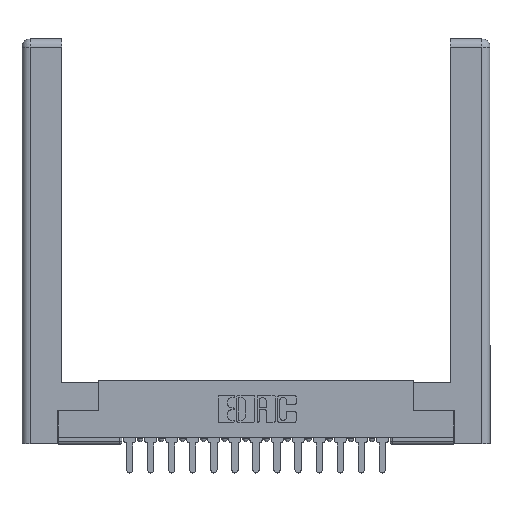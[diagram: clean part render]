
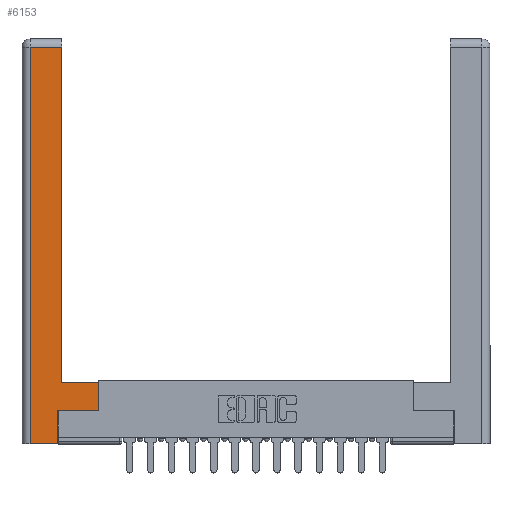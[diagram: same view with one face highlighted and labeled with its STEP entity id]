
A CAD part, top view. The second image highlights one B-rep face of the part: STEP entity #6153.
In plain terms, the highlighted planar face has unit normal (0, 0, 1).
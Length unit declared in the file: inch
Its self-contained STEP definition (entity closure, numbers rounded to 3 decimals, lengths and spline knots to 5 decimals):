
#14 = ORIENTED_EDGE ( 'NONE', *, *, #15030, .T. ) ;
#249 = DIRECTION ( 'NONE',  ( 0., 1., 0. ) ) ;
#354 = CARTESIAN_POINT ( 'NONE',  ( 0.565, 0.245, 0. ) ) ;
#395 = ORIENTED_EDGE ( 'NONE', *, *, #15939, .T. ) ;
#446 = PLANE ( 'NONE',  #3961 ) ;
#534 = DIRECTION ( 'NONE',  ( 0., 0., -1. ) ) ;
#678 = ORIENTED_EDGE ( 'NONE', *, *, #12717, .T. ) ;
#901 = ORIENTED_EDGE ( 'NONE', *, *, #13060, .T. ) ;
#1120 = DIRECTION ( 'NONE',  ( -1., 0., 0. ) ) ;
#1515 = DIRECTION ( 'NONE',  ( 0., 1., 0. ) ) ;
#1787 = FACE_OUTER_BOUND ( 'NONE', #15065, .T. ) ;
#2013 = CARTESIAN_POINT ( 'NONE',  ( 0.295, 3., 0. ) ) ;
#2034 = VERTEX_POINT ( 'NONE', #11718 ) ;
#2072 = CARTESIAN_POINT ( 'NONE',  ( 0.265, 0.245, 0. ) ) ;
#2492 = DIRECTION ( 'NONE',  ( 1., 0., 0. ) ) ;
#2724 = DIRECTION ( 'NONE',  ( -1., 0., 0. ) ) ;
#3560 = VERTEX_POINT ( 'NONE', #7388 ) ;
#3961 = AXIS2_PLACEMENT_3D ( 'NONE', #12844, #534, #8792 ) ;
#4356 = DIRECTION ( 'NONE',  ( 0., 1., 0. ) ) ;
#4361 = EDGE_CURVE ( 'NONE', #13816, #15990, #12673, .T. ) ;
#4656 = VECTOR ( 'NONE', #7862, 39.37008 ) ;
#4718 = CARTESIAN_POINT ( 'NONE',  ( 0.0615, 2.94, 0. ) ) ;
#5055 = LINE ( 'NONE', #14759, #6821 ) ;
#5098 = CARTESIAN_POINT ( 'NONE',  ( 0.565, 0.245, 0. ) ) ;
#5259 = CARTESIAN_POINT ( 'NONE',  ( 0.265, 0., 0. ) ) ;
#5339 = VERTEX_POINT ( 'NONE', #2072 ) ;
#6153 = ADVANCED_FACE ( 'NONE', ( #1787 ), #446, .F. ) ;
#6733 = LINE ( 'NONE', #5098, #16855 ) ;
#6821 = VECTOR ( 'NONE', #1120, 39.37008 ) ;
#7144 = ORIENTED_EDGE ( 'NONE', *, *, #4361, .T. ) ;
#7369 = CARTESIAN_POINT ( 'NONE',  ( 0.265, 0., 0. ) ) ;
#7388 = CARTESIAN_POINT ( 'NONE',  ( 0.295, 0.45, 0. ) ) ;
#7862 = DIRECTION ( 'NONE',  ( 1., 0., 0. ) ) ;
#7930 = LINE ( 'NONE', #8114, #17191 ) ;
#7995 = EDGE_CURVE ( 'NONE', #14933, #5339, #15332, .T. ) ;
#8114 = CARTESIAN_POINT ( 'NONE',  ( 0.295, 0.45, 0. ) ) ;
#8703 = EDGE_CURVE ( 'NONE', #15990, #3560, #7930, .T. ) ;
#8723 = ORIENTED_EDGE ( 'NONE', *, *, #8703, .T. ) ;
#8792 = DIRECTION ( 'NONE',  ( -1., 0., 0. ) ) ;
#9548 = DIRECTION ( 'NONE',  ( 0., -1., 0. ) ) ;
#9633 = CARTESIAN_POINT ( 'NONE',  ( 0.565, 0.45, 0. ) ) ;
#9909 = CARTESIAN_POINT ( 'NONE',  ( 0.0615, 0., 0. ) ) ;
#9924 = LINE ( 'NONE', #2013, #14201 ) ;
#10494 = VECTOR ( 'NONE', #1515, 39.37008 ) ;
#11470 = CARTESIAN_POINT ( 'NONE',  ( 0.265, 0.245, 0. ) ) ;
#11718 = CARTESIAN_POINT ( 'NONE',  ( 0.295, 2.94, 0. ) ) ;
#12673 = LINE ( 'NONE', #16701, #10494 ) ;
#12717 = EDGE_CURVE ( 'NONE', #13545, #14933, #13271, .T. ) ;
#12844 = CARTESIAN_POINT ( 'NONE',  ( 0., 0., 0. ) ) ;
#12895 = ORIENTED_EDGE ( 'NONE', *, *, #7995, .T. ) ;
#13025 = ORIENTED_EDGE ( 'NONE', *, *, #17240, .T. ) ;
#13060 = EDGE_CURVE ( 'NONE', #3560, #2034, #9924, .T. ) ;
#13271 = LINE ( 'NONE', #5259, #4656 ) ;
#13450 = VECTOR ( 'NONE', #249, 39.37008 ) ;
#13545 = VERTEX_POINT ( 'NONE', #9909 ) ;
#13816 = VERTEX_POINT ( 'NONE', #354 ) ;
#14201 = VECTOR ( 'NONE', #4356, 39.37008 ) ;
#14759 = CARTESIAN_POINT ( 'NONE',  ( 0.0615, 2.94, 0. ) ) ;
#14824 = CARTESIAN_POINT ( 'NONE',  ( 0.0615, 0., 0. ) ) ;
#14853 = VECTOR ( 'NONE', #9548, 39.37008 ) ;
#14933 = VERTEX_POINT ( 'NONE', #7369 ) ;
#15030 = EDGE_CURVE ( 'NONE', #5339, #13816, #6733, .T. ) ;
#15065 = EDGE_LOOP ( 'NONE', ( #901, #13025, #395, #678, #12895, #14, #7144, #8723 ) ) ;
#15305 = VERTEX_POINT ( 'NONE', #4718 ) ;
#15332 = LINE ( 'NONE', #11470, #13450 ) ;
#15939 = EDGE_CURVE ( 'NONE', #15305, #13545, #16276, .T. ) ;
#15990 = VERTEX_POINT ( 'NONE', #9633 ) ;
#16276 = LINE ( 'NONE', #14824, #14853 ) ;
#16701 = CARTESIAN_POINT ( 'NONE',  ( 0.565, 0.45, 0. ) ) ;
#16855 = VECTOR ( 'NONE', #2492, 39.37008 ) ;
#17191 = VECTOR ( 'NONE', #2724, 39.37008 ) ;
#17240 = EDGE_CURVE ( 'NONE', #2034, #15305, #5055, .T. ) ;
